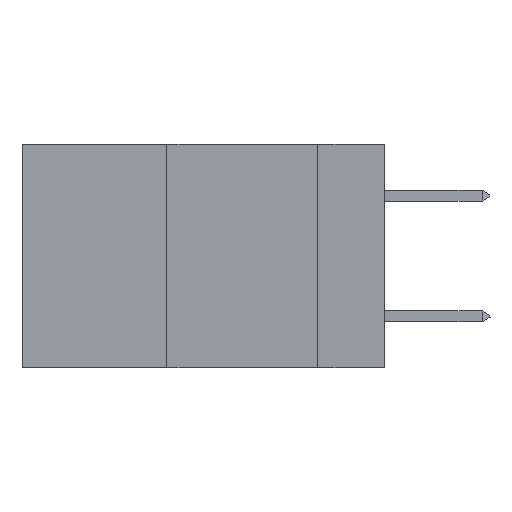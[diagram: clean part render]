
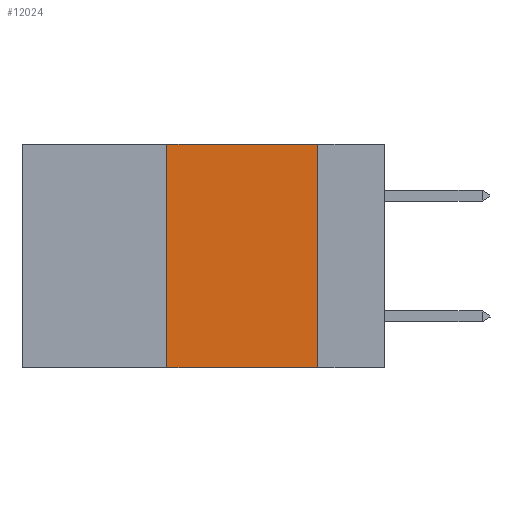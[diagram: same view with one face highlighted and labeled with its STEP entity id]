
A CAD part, left-side view. The second image highlights one B-rep face of the part: STEP entity #12024.
In plain terms, the highlighted planar face has unit normal (-1, 0, 0).
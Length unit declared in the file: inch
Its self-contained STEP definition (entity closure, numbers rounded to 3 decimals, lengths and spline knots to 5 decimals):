
#801 = ORIENTED_EDGE ( 'NONE', *, *, #2168, .F. ) ;
#1529 = PLANE ( 'NONE',  #7651 ) ;
#1556 = EDGE_CURVE ( 'NONE', #4109, #8267, #2346, .T. ) ;
#1639 = DIRECTION ( 'NONE',  ( 0., -1., 0. ) ) ;
#1844 = DIRECTION ( 'NONE',  ( 0., 0., 1. ) ) ;
#1899 = LINE ( 'NONE', #11150, #4310 ) ;
#2168 = EDGE_CURVE ( 'NONE', #7523, #4109, #3456, .T. ) ;
#2346 = LINE ( 'NONE', #3868, #9642 ) ;
#2359 = LINE ( 'NONE', #8161, #4050 ) ;
#2676 = DIRECTION ( 'NONE',  ( 0., 0., -1. ) ) ;
#2730 = CARTESIAN_POINT ( 'NONE',  ( 0., 0.6, 0. ) ) ;
#3456 = LINE ( 'NONE', #2730, #7557 ) ;
#3868 = CARTESIAN_POINT ( 'NONE',  ( 0., 0.11, 0. ) ) ;
#4050 = VECTOR ( 'NONE', #1844, 39.37008 ) ;
#4077 = CARTESIAN_POINT ( 'NONE',  ( 0., 0.36, 0. ) ) ;
#4109 = VERTEX_POINT ( 'NONE', #9231 ) ;
#4310 = VECTOR ( 'NONE', #12431, 39.37008 ) ;
#4391 = CARTESIAN_POINT ( 'NONE',  ( 0., 0.11, -0.37 ) ) ;
#5574 = VERTEX_POINT ( 'NONE', #9702 ) ;
#7523 = VERTEX_POINT ( 'NONE', #4077 ) ;
#7557 = VECTOR ( 'NONE', #1639, 39.37008 ) ;
#7651 = AXIS2_PLACEMENT_3D ( 'NONE', #10955, #11131, #2676 ) ;
#7685 = DIRECTION ( 'NONE',  ( 0., 0., -1. ) ) ;
#8161 = CARTESIAN_POINT ( 'NONE',  ( 0., 0.36, 0. ) ) ;
#8267 = VERTEX_POINT ( 'NONE', #4391 ) ;
#8570 = FACE_OUTER_BOUND ( 'NONE', #13831, .T. ) ;
#8610 = ORIENTED_EDGE ( 'NONE', *, *, #13144, .F. ) ;
#9231 = CARTESIAN_POINT ( 'NONE',  ( 0., 0.11, 0. ) ) ;
#9642 = VECTOR ( 'NONE', #7685, 39.37008 ) ;
#9702 = CARTESIAN_POINT ( 'NONE',  ( 0., 0.36, -0.37 ) ) ;
#10165 = ORIENTED_EDGE ( 'NONE', *, *, #10766, .T. ) ;
#10766 = EDGE_CURVE ( 'NONE', #5574, #8267, #1899, .T. ) ;
#10955 = CARTESIAN_POINT ( 'NONE',  ( 0., 0.6, 0. ) ) ;
#11131 = DIRECTION ( 'NONE',  ( 1., 0., 0. ) ) ;
#11150 = CARTESIAN_POINT ( 'NONE',  ( 0., 0.6, -0.37 ) ) ;
#12024 = ADVANCED_FACE ( 'NONE', ( #8570 ), #1529, .F. ) ;
#12431 = DIRECTION ( 'NONE',  ( 0., -1., 0. ) ) ;
#13073 = ORIENTED_EDGE ( 'NONE', *, *, #1556, .F. ) ;
#13144 = EDGE_CURVE ( 'NONE', #5574, #7523, #2359, .T. ) ;
#13831 = EDGE_LOOP ( 'NONE', ( #13073, #801, #8610, #10165 ) ) ;
